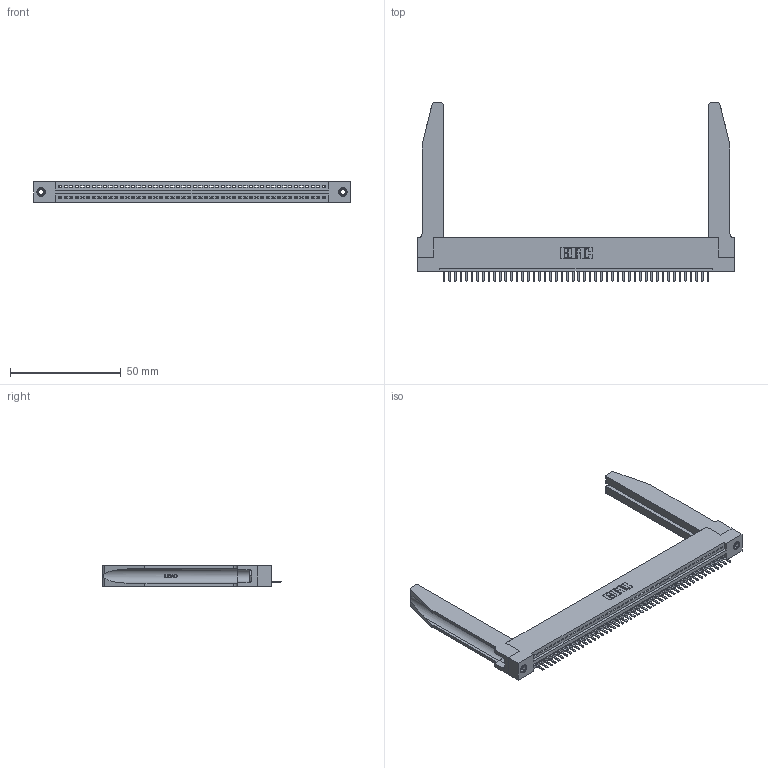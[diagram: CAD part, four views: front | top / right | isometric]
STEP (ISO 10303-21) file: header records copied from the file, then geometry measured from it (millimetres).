
FILE_DESCRIPTION (( 'STEP AP203' ), '1' );
FILE_NAME ('345-048-520-178.STEP', '2019-10-09T04:06:08', ( '' ), ( '' ), 'SwSTEP 2.0', 'SolidWorks 2016', '' );
FILE_SCHEMA (( 'CONFIG_CONTROL_DESIGN' ));
Length unit declared in the file: inch
Products named in the file (5): 345-292-001_345-293-120; 345-250-001_345-250-001-102; 345 Part_Flush Mounting Lugs - 0.156 Dia-TH; 345-048-520-178; 345-220-078_345-220-078
Assembly tree (53 placements, depth 2):
  345-048-520-178
    345 Part_Flush Mounting Lugs - 0.156 Dia-TH
    345-292-001_345-293-120  x48
    345-250-001_345-250-001-102  x2
    345-220-078_345-220-078  x2
Bounding box: 143.15 x 80.64 x 9.4 mm (x, y, z)
Volume: 21278.5 mm3; surface area: 24426.4 mm2
Topology: 53 solids, 53 shells, 3336 faces, 9781 edges, 6382 vertices
Faces by surface type: plane 2238, cylinder 1046, bspline 36, cone 12, torus 4
Entity records: 40172 total; most frequent: CARTESIAN_POINT 7867, ORIENTED_EDGE 6734, DIRECTION 5857, EDGE_CURVE 3367, VECTOR 2945, LINE 2945, VERTEX_POINT 2236, AXIS2_PLACEMENT_3D 1456
